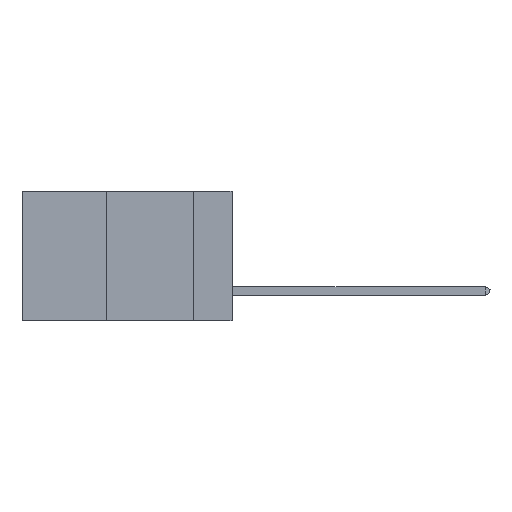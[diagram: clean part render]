
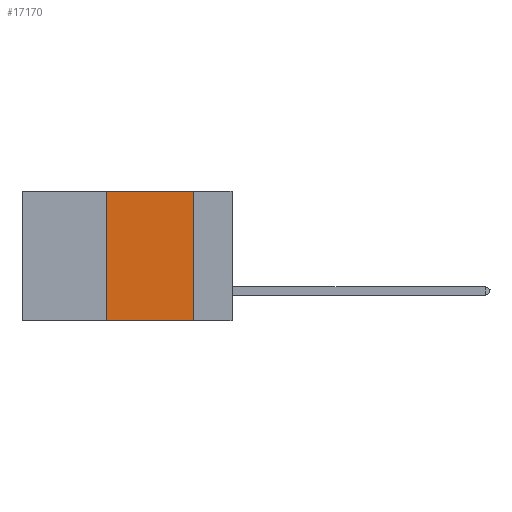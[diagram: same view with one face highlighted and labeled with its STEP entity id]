
A CAD part, left-side view. The second image highlights one B-rep face of the part: STEP entity #17170.
In plain terms, the highlighted planar face has unit normal (-1, 0, 0).
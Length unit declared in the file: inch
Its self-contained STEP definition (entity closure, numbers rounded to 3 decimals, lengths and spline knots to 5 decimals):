
#715 = LINE ( 'NONE', #46415, #29456 ) ;
#2877 = CARTESIAN_POINT ( 'NONE',  ( 0., 0.6, 0. ) ) ;
#3301 = VECTOR ( 'NONE', #7406, 39.37008 ) ;
#6722 = DIRECTION ( 'NONE',  ( 0., 0., -1. ) ) ;
#7406 = DIRECTION ( 'NONE',  ( 0., 0., -1. ) ) ;
#8200 = LINE ( 'NONE', #29628, #16606 ) ;
#9098 = CARTESIAN_POINT ( 'NONE',  ( 0., 0.36, 0. ) ) ;
#10265 = PLANE ( 'NONE',  #33209 ) ;
#10430 = DIRECTION ( 'NONE',  ( 1., 0., 0. ) ) ;
#11604 = DIRECTION ( 'NONE',  ( 0., 0., 1. ) ) ;
#14109 = ORIENTED_EDGE ( 'NONE', *, *, #33566, .F. ) ;
#15842 = VERTEX_POINT ( 'NONE', #36989 ) ;
#16606 = VECTOR ( 'NONE', #18223, 39.37008 ) ;
#17170 = ADVANCED_FACE ( 'NONE', ( #48036 ), #10265, .F. ) ;
#18128 = CARTESIAN_POINT ( 'NONE',  ( 0., 0.11, 0. ) ) ;
#18223 = DIRECTION ( 'NONE',  ( 0., -1., 0. ) ) ;
#19175 = VECTOR ( 'NONE', #11604, 39.37008 ) ;
#19431 = LINE ( 'NONE', #30493, #3301 ) ;
#19826 = VERTEX_POINT ( 'NONE', #9098 ) ;
#20072 = ORIENTED_EDGE ( 'NONE', *, *, #26408, .T. ) ;
#23311 = VERTEX_POINT ( 'NONE', #18128 ) ;
#24231 = VERTEX_POINT ( 'NONE', #38980 ) ;
#26408 = EDGE_CURVE ( 'NONE', #24231, #15842, #8200, .T. ) ;
#26634 = CARTESIAN_POINT ( 'NONE',  ( 0., 0.36, 0. ) ) ;
#29456 = VECTOR ( 'NONE', #42403, 39.37008 ) ;
#29628 = CARTESIAN_POINT ( 'NONE',  ( 0., 0.6, -0.37 ) ) ;
#30075 = EDGE_CURVE ( 'NONE', #19826, #23311, #715, .T. ) ;
#30333 = ORIENTED_EDGE ( 'NONE', *, *, #30678, .F. ) ;
#30493 = CARTESIAN_POINT ( 'NONE',  ( 0., 0.11, 0. ) ) ;
#30678 = EDGE_CURVE ( 'NONE', #24231, #19826, #34753, .T. ) ;
#31434 = EDGE_LOOP ( 'NONE', ( #14109, #35342, #30333, #20072 ) ) ;
#33209 = AXIS2_PLACEMENT_3D ( 'NONE', #2877, #10430, #6722 ) ;
#33566 = EDGE_CURVE ( 'NONE', #23311, #15842, #19431, .T. ) ;
#34753 = LINE ( 'NONE', #26634, #19175 ) ;
#35342 = ORIENTED_EDGE ( 'NONE', *, *, #30075, .F. ) ;
#36989 = CARTESIAN_POINT ( 'NONE',  ( 0., 0.11, -0.37 ) ) ;
#38980 = CARTESIAN_POINT ( 'NONE',  ( 0., 0.36, -0.37 ) ) ;
#42403 = DIRECTION ( 'NONE',  ( 0., -1., 0. ) ) ;
#46415 = CARTESIAN_POINT ( 'NONE',  ( 0., 0.6, 0. ) ) ;
#48036 = FACE_OUTER_BOUND ( 'NONE', #31434, .T. ) ;
